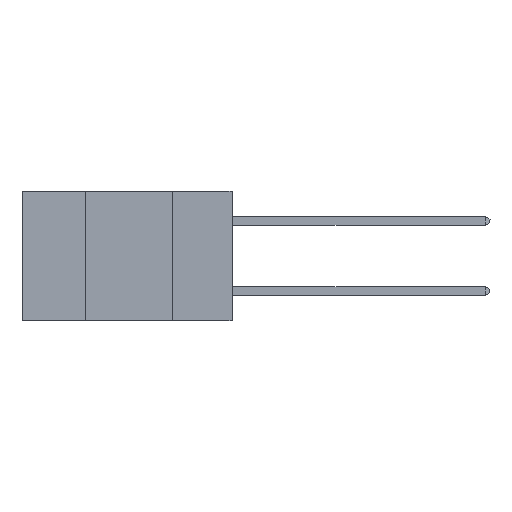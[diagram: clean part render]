
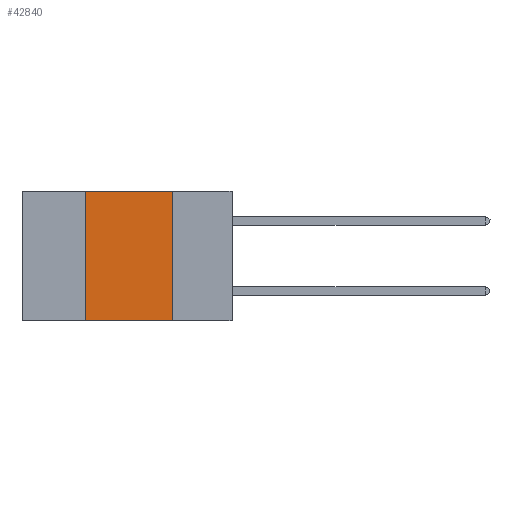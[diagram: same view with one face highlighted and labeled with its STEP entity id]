
A CAD part, left-side view. The second image highlights one B-rep face of the part: STEP entity #42840.
In plain terms, the highlighted planar face has unit normal (-1, 0, 0).
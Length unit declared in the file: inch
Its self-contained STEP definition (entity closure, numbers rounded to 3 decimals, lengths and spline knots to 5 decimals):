
#639 = CARTESIAN_POINT ( 'NONE',  ( 0., 0.17, 0. ) ) ;
#2159 = CARTESIAN_POINT ( 'NONE',  ( 0., 0.42, -0.37 ) ) ;
#3543 = CARTESIAN_POINT ( 'NONE',  ( 0., 0.17, 0. ) ) ;
#4277 = EDGE_CURVE ( 'NONE', #14513, #4671, #11216, .T. ) ;
#4671 = VERTEX_POINT ( 'NONE', #3543 ) ;
#4746 = EDGE_CURVE ( 'NONE', #4671, #7734, #24677, .T. ) ;
#7187 = DIRECTION ( 'NONE',  ( 0., -1., 0. ) ) ;
#7734 = VERTEX_POINT ( 'NONE', #43598 ) ;
#9141 = AXIS2_PLACEMENT_3D ( 'NONE', #37927, #37702, #41319 ) ;
#11216 = LINE ( 'NONE', #21353, #22324 ) ;
#12789 = ORIENTED_EDGE ( 'NONE', *, *, #19390, .T. ) ;
#13667 = ORIENTED_EDGE ( 'NONE', *, *, #4277, .F. ) ;
#13956 = LINE ( 'NONE', #28306, #43102 ) ;
#14176 = DIRECTION ( 'NONE',  ( 0., -1., 0. ) ) ;
#14513 = VERTEX_POINT ( 'NONE', #21906 ) ;
#15353 = EDGE_LOOP ( 'NONE', ( #21348, #13667, #28116, #12789 ) ) ;
#16809 = PLANE ( 'NONE',  #9141 ) ;
#17932 = CARTESIAN_POINT ( 'NONE',  ( 0., 0.42, 0. ) ) ;
#19390 = EDGE_CURVE ( 'NONE', #40801, #7734, #13956, .T. ) ;
#21348 = ORIENTED_EDGE ( 'NONE', *, *, #4746, .F. ) ;
#21353 = CARTESIAN_POINT ( 'NONE',  ( 0., 0.6, 0. ) ) ;
#21906 = CARTESIAN_POINT ( 'NONE',  ( 0., 0.42, 0. ) ) ;
#22324 = VECTOR ( 'NONE', #7187, 39.37008 ) ;
#24044 = EDGE_CURVE ( 'NONE', #40801, #14513, #24693, .T. ) ;
#24677 = LINE ( 'NONE', #639, #30289 ) ;
#24693 = LINE ( 'NONE', #17932, #33205 ) ;
#28116 = ORIENTED_EDGE ( 'NONE', *, *, #24044, .F. ) ;
#28306 = CARTESIAN_POINT ( 'NONE',  ( 0., 0.6, -0.37 ) ) ;
#30289 = VECTOR ( 'NONE', #42211, 39.37008 ) ;
#33205 = VECTOR ( 'NONE', #38401, 39.37008 ) ;
#37702 = DIRECTION ( 'NONE',  ( 1., 0., 0. ) ) ;
#37927 = CARTESIAN_POINT ( 'NONE',  ( 0., 0.6, 0. ) ) ;
#38401 = DIRECTION ( 'NONE',  ( 0., 0., 1. ) ) ;
#40801 = VERTEX_POINT ( 'NONE', #2159 ) ;
#41319 = DIRECTION ( 'NONE',  ( 0., 0., -1. ) ) ;
#41542 = FACE_OUTER_BOUND ( 'NONE', #15353, .T. ) ;
#42211 = DIRECTION ( 'NONE',  ( 0., 0., -1. ) ) ;
#42840 = ADVANCED_FACE ( 'NONE', ( #41542 ), #16809, .F. ) ;
#43102 = VECTOR ( 'NONE', #14176, 39.37008 ) ;
#43598 = CARTESIAN_POINT ( 'NONE',  ( 0., 0.17, -0.37 ) ) ;
